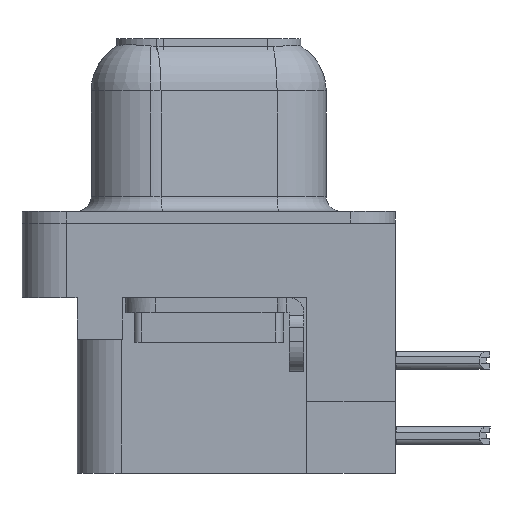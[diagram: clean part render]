
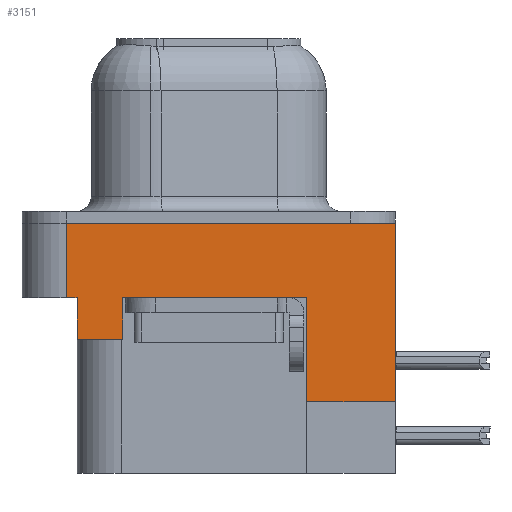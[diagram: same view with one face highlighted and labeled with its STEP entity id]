
A CAD part, left-side view. The second image highlights one B-rep face of the part: STEP entity #3151.
In plain terms, the highlighted planar face has unit normal (-1, 0, 0).
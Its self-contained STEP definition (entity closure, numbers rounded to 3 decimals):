
#383 = VERTEX_POINT ( 'NONE', #2462 ) ;
#625 = EDGE_LOOP ( 'NONE', ( #9639, #1375, #1371, #20121, #11501, #21112, #21047, #1131, #3550, #3819 ) ) ;
#711 = EDGE_CURVE ( 'NONE', #13724, #22675, #15803, .T. ) ;
#990 = CARTESIAN_POINT ( 'NONE',  ( -2.935, 4.775, -2.5 ) ) ;
#1131 = ORIENTED_EDGE ( 'NONE', *, *, #7414, .T. ) ;
#1157 = VECTOR ( 'NONE', #15666, 1000. ) ;
#1371 = ORIENTED_EDGE ( 'NONE', *, *, #711, .F. ) ;
#1375 = ORIENTED_EDGE ( 'NONE', *, *, #7788, .T. ) ;
#1413 = DIRECTION ( 'NONE',  ( 0., 1., 0. ) ) ;
#1855 = CARTESIAN_POINT ( 'NONE',  ( -2.935, 2.895, -3.9 ) ) ;
#2276 = LINE ( 'NONE', #1855, #21068 ) ;
#2462 = CARTESIAN_POINT ( 'NONE',  ( -2.935, 2.895, -2.5 ) ) ;
#2774 = CARTESIAN_POINT ( 'NONE',  ( -2.935, -6.275, 0. ) ) ;
#3151 = ADVANCED_FACE ( 'NONE', ( #3281 ), #15949, .T. ) ;
#3281 = FACE_OUTER_BOUND ( 'NONE', #625, .T. ) ;
#3463 = LINE ( 'NONE', #21058, #1157 ) ;
#3550 = ORIENTED_EDGE ( 'NONE', *, *, #14493, .T. ) ;
#3714 = DIRECTION ( 'NONE',  ( 0., 0., 1. ) ) ;
#3819 = ORIENTED_EDGE ( 'NONE', *, *, #13767, .F. ) ;
#5140 = DIRECTION ( 'NONE',  ( -1., 0., 0. ) ) ;
#5904 = DIRECTION ( 'NONE',  ( 0., -1., 0. ) ) ;
#5921 = EDGE_CURVE ( 'NONE', #18510, #9457, #3463, .T. ) ;
#6040 = EDGE_CURVE ( 'NONE', #19589, #16305, #9201, .T. ) ;
#6769 = LINE ( 'NONE', #8728, #11027 ) ;
#7414 = EDGE_CURVE ( 'NONE', #19589, #383, #2276, .T. ) ;
#7788 = EDGE_CURVE ( 'NONE', #18510, #22675, #10009, .T. ) ;
#8111 = LINE ( 'NONE', #9769, #17727 ) ;
#8271 = DIRECTION ( 'NONE',  ( 0., 0., 1. ) ) ;
#8559 = CARTESIAN_POINT ( 'NONE',  ( -2.935, -3.295, -2.5 ) ) ;
#8728 = CARTESIAN_POINT ( 'NONE',  ( -2.935, 4.425, -3.9 ) ) ;
#9201 = LINE ( 'NONE', #21460, #13437 ) ;
#9457 = VERTEX_POINT ( 'NONE', #16181 ) ;
#9639 = ORIENTED_EDGE ( 'NONE', *, *, #5921, .F. ) ;
#9769 = CARTESIAN_POINT ( 'NONE',  ( -2.935, -3.295, -8.4 ) ) ;
#10009 = LINE ( 'NONE', #17281, #15371 ) ;
#10048 = LINE ( 'NONE', #19380, #19104 ) ;
#10270 = VERTEX_POINT ( 'NONE', #13060 ) ;
#10337 = CARTESIAN_POINT ( 'NONE',  ( -2.935, -6.275, -6. ) ) ;
#10367 = CARTESIAN_POINT ( 'NONE',  ( -2.935, 4.425, -3.9 ) ) ;
#11018 = VECTOR ( 'NONE', #17514, 1000. ) ;
#11027 = VECTOR ( 'NONE', #19569, 1000. ) ;
#11357 = VERTEX_POINT ( 'NONE', #8559 ) ;
#11501 = ORIENTED_EDGE ( 'NONE', *, *, #11720, .T. ) ;
#11592 = AXIS2_PLACEMENT_3D ( 'NONE', #19600, #5140, #17849 ) ;
#11720 = EDGE_CURVE ( 'NONE', #17476, #10270, #23496, .T. ) ;
#11988 = DIRECTION ( 'NONE',  ( 0., 0., 1. ) ) ;
#13060 = CARTESIAN_POINT ( 'NONE',  ( -2.935, 4.425, -2.5 ) ) ;
#13437 = VECTOR ( 'NONE', #1413, 1000. ) ;
#13518 = CARTESIAN_POINT ( 'NONE',  ( -2.935, 2.895, -3.9 ) ) ;
#13724 = VERTEX_POINT ( 'NONE', #20469 ) ;
#13767 = EDGE_CURVE ( 'NONE', #9457, #11357, #8111, .T. ) ;
#14493 = EDGE_CURVE ( 'NONE', #383, #11357, #10048, .T. ) ;
#14809 = CARTESIAN_POINT ( 'NONE',  ( -2.935, -6.275, 0. ) ) ;
#15371 = VECTOR ( 'NONE', #8271, 1000. ) ;
#15666 = DIRECTION ( 'NONE',  ( 0., 1., 0. ) ) ;
#15803 = LINE ( 'NONE', #14809, #11018 ) ;
#15949 = PLANE ( 'NONE',  #11592 ) ;
#16181 = CARTESIAN_POINT ( 'NONE',  ( -2.935, -3.295, -6. ) ) ;
#16305 = VERTEX_POINT ( 'NONE', #10367 ) ;
#16888 = EDGE_CURVE ( 'NONE', #17476, #13724, #17314, .T. ) ;
#17281 = CARTESIAN_POINT ( 'NONE',  ( -2.935, -6.275, -2.5 ) ) ;
#17314 = LINE ( 'NONE', #17364, #21584 ) ;
#17364 = CARTESIAN_POINT ( 'NONE',  ( -2.935, 4.775, -2.5 ) ) ;
#17476 = VERTEX_POINT ( 'NONE', #990 ) ;
#17514 = DIRECTION ( 'NONE',  ( 0., -1., 0. ) ) ;
#17727 = VECTOR ( 'NONE', #22444, 1000. ) ;
#17849 = DIRECTION ( 'NONE',  ( 0., 0., 1. ) ) ;
#18510 = VERTEX_POINT ( 'NONE', #10337 ) ;
#18511 = CARTESIAN_POINT ( 'NONE',  ( -2.935, -6.275, -2.5 ) ) ;
#18651 = VECTOR ( 'NONE', #5904, 1000. ) ;
#19104 = VECTOR ( 'NONE', #21189, 1000. ) ;
#19212 = EDGE_CURVE ( 'NONE', #16305, #10270, #6769, .T. ) ;
#19380 = CARTESIAN_POINT ( 'NONE',  ( -2.935, -6.275, -2.5 ) ) ;
#19569 = DIRECTION ( 'NONE',  ( 0., 0., 1. ) ) ;
#19589 = VERTEX_POINT ( 'NONE', #13518 ) ;
#19600 = CARTESIAN_POINT ( 'NONE',  ( -2.935, -6.275, -2.5 ) ) ;
#20121 = ORIENTED_EDGE ( 'NONE', *, *, #16888, .F. ) ;
#20469 = CARTESIAN_POINT ( 'NONE',  ( -2.935, 4.775, 0. ) ) ;
#21047 = ORIENTED_EDGE ( 'NONE', *, *, #6040, .F. ) ;
#21058 = CARTESIAN_POINT ( 'NONE',  ( -2.935, -6.495, -6. ) ) ;
#21068 = VECTOR ( 'NONE', #3714, 1000. ) ;
#21112 = ORIENTED_EDGE ( 'NONE', *, *, #19212, .F. ) ;
#21189 = DIRECTION ( 'NONE',  ( 0., -1., 0. ) ) ;
#21460 = CARTESIAN_POINT ( 'NONE',  ( -2.935, 4.425, -3.9 ) ) ;
#21584 = VECTOR ( 'NONE', #11988, 1000. ) ;
#22444 = DIRECTION ( 'NONE',  ( 0., 0., 1. ) ) ;
#22675 = VERTEX_POINT ( 'NONE', #2774 ) ;
#23496 = LINE ( 'NONE', #18511, #18651 ) ;
